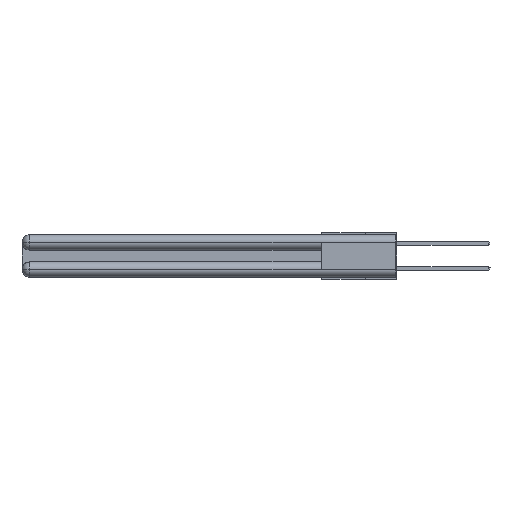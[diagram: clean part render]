
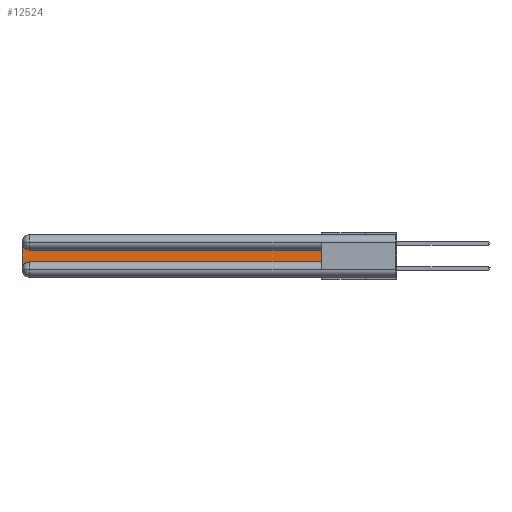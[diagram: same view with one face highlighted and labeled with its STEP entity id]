
A CAD part, left-side view. The second image highlights one B-rep face of the part: STEP entity #12524.
In plain terms, the highlighted planar face has unit normal (-1, 0, 0).
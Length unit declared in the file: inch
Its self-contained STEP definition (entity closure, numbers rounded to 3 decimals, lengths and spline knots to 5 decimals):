
#4 = EDGE_CURVE ( 'NONE', #16196, #27000, #18506, .T. ) ;
#136 = LINE ( 'NONE', #6000, #17489 ) ;
#423 = DIRECTION ( 'NONE',  ( 0., 0., -1. ) ) ;
#2757 = DIRECTION ( 'NONE',  ( 1., 0., 0. ) ) ;
#2891 = AXIS2_PLACEMENT_3D ( 'NONE', #26329, #16650, #423 ) ;
#3447 = VECTOR ( 'NONE', #15545, 39.37008 ) ;
#3625 = DIRECTION ( 'NONE',  ( 0., 0., -1. ) ) ;
#3983 = ORIENTED_EDGE ( 'NONE', *, *, #20804, .T. ) ;
#4006 = VERTEX_POINT ( 'NONE', #24953 ) ;
#4919 = EDGE_CURVE ( 'NONE', #7424, #4006, #10619, .T. ) ;
#5526 = CARTESIAN_POINT ( 'NONE',  ( 0.075, 3., -0.0625 ) ) ;
#6000 = CARTESIAN_POINT ( 'NONE',  ( 0.075, 3., -0.2175 ) ) ;
#6007 = CARTESIAN_POINT ( 'NONE',  ( 0.075, 2.94, -0.2775 ) ) ;
#6772 = CARTESIAN_POINT ( 'NONE',  ( 0.075, 3., -0.2775 ) ) ;
#7424 = VERTEX_POINT ( 'NONE', #30516 ) ;
#8555 = EDGE_LOOP ( 'NONE', ( #25377, #20793, #24461, #17098, #3983, #17453 ) ) ;
#8662 = EDGE_CURVE ( 'NONE', #13862, #16196, #136, .T. ) ;
#8938 = CARTESIAN_POINT ( 'NONE',  ( 0.075, 0.6, -0.1225 ) ) ;
#10619 = LINE ( 'NONE', #8938, #23873 ) ;
#11464 = CARTESIAN_POINT ( 'NONE',  ( 0.075, 0.6, -0.2175 ) ) ;
#12524 = ADVANCED_FACE ( 'NONE', ( #16016 ), #28393, .F. ) ;
#13695 = CIRCLE ( 'NONE', #2891, 0.06 ) ;
#13862 = VERTEX_POINT ( 'NONE', #5526 ) ;
#14265 = CARTESIAN_POINT ( 'NONE',  ( 0.075, 3., -0.1225 ) ) ;
#14448 = VERTEX_POINT ( 'NONE', #11464 ) ;
#15170 = DIRECTION ( 'NONE',  ( 1., 0., 0. ) ) ;
#15331 = CARTESIAN_POINT ( 'NONE',  ( 0.075, 0.6, -0.2175 ) ) ;
#15545 = DIRECTION ( 'NONE',  ( 0., 0., 1. ) ) ;
#16016 = FACE_OUTER_BOUND ( 'NONE', #8555, .T. ) ;
#16196 = VERTEX_POINT ( 'NONE', #6772 ) ;
#16650 = DIRECTION ( 'NONE',  ( 1., 0., 0. ) ) ;
#17098 = ORIENTED_EDGE ( 'NONE', *, *, #4, .T. ) ;
#17453 = ORIENTED_EDGE ( 'NONE', *, *, #24391, .T. ) ;
#17489 = VECTOR ( 'NONE', #3625, 39.37008 ) ;
#17651 = DIRECTION ( 'NONE',  ( 0., 0., -1. ) ) ;
#18506 = CIRCLE ( 'NONE', #26385, 0.06 ) ;
#19996 = LINE ( 'NONE', #29190, #21535 ) ;
#20793 = ORIENTED_EDGE ( 'NONE', *, *, #29612, .T. ) ;
#20804 = EDGE_CURVE ( 'NONE', #27000, #14448, #19996, .T. ) ;
#21535 = VECTOR ( 'NONE', #22173, 39.37008 ) ;
#22173 = DIRECTION ( 'NONE',  ( 0., -1., 0. ) ) ;
#23873 = VECTOR ( 'NONE', #27759, 39.37008 ) ;
#24391 = EDGE_CURVE ( 'NONE', #14448, #7424, #28851, .T. ) ;
#24461 = ORIENTED_EDGE ( 'NONE', *, *, #8662, .T. ) ;
#24953 = CARTESIAN_POINT ( 'NONE',  ( 0.075, 2.94, -0.1225 ) ) ;
#25377 = ORIENTED_EDGE ( 'NONE', *, *, #4919, .T. ) ;
#26329 = CARTESIAN_POINT ( 'NONE',  ( 0.075, 2.94, -0.0625 ) ) ;
#26385 = AXIS2_PLACEMENT_3D ( 'NONE', #6007, #15170, #17651 ) ;
#27000 = VERTEX_POINT ( 'NONE', #29467 ) ;
#27759 = DIRECTION ( 'NONE',  ( 0., 1., 0. ) ) ;
#28393 = PLANE ( 'NONE',  #29647 ) ;
#28599 = DIRECTION ( 'NONE',  ( 0., 0., -1. ) ) ;
#28851 = LINE ( 'NONE', #15331, #3447 ) ;
#29190 = CARTESIAN_POINT ( 'NONE',  ( 0.075, 0.6, -0.2175 ) ) ;
#29467 = CARTESIAN_POINT ( 'NONE',  ( 0.075, 2.94, -0.2175 ) ) ;
#29612 = EDGE_CURVE ( 'NONE', #4006, #13862, #13695, .T. ) ;
#29647 = AXIS2_PLACEMENT_3D ( 'NONE', #14265, #2757, #28599 ) ;
#30516 = CARTESIAN_POINT ( 'NONE',  ( 0.075, 0.6, -0.1225 ) ) ;
